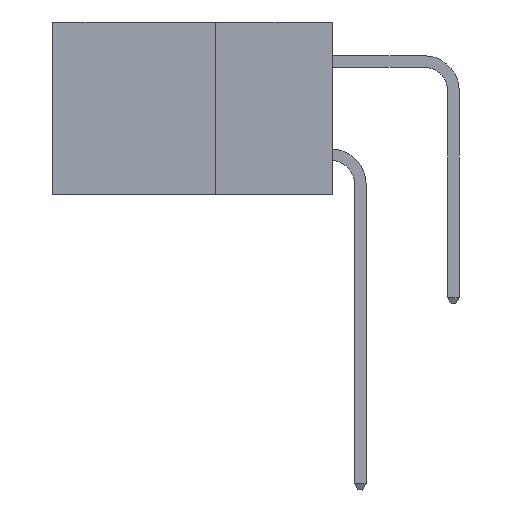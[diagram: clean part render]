
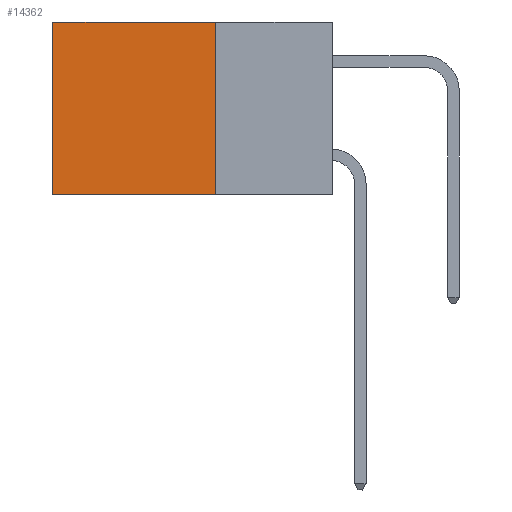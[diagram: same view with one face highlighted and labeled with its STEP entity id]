
A CAD part, left-side view. The second image highlights one B-rep face of the part: STEP entity #14362.
In plain terms, the highlighted planar face has unit normal (-1, 0, 0).
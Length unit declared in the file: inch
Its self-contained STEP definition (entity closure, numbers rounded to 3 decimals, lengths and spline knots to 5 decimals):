
#1033 = LINE ( 'NONE', #18068, #15423 ) ;
#1094 = VERTEX_POINT ( 'NONE', #8958 ) ;
#2006 = AXIS2_PLACEMENT_3D ( 'NONE', #20514, #6875, #14598 ) ;
#4062 = LINE ( 'NONE', #20553, #10786 ) ;
#6875 = DIRECTION ( 'NONE',  ( 1., 0., 0. ) ) ;
#6929 = VERTEX_POINT ( 'NONE', #7179 ) ;
#7179 = CARTESIAN_POINT ( 'NONE',  ( 0.298, 0.25, 0. ) ) ;
#7870 = DIRECTION ( 'NONE',  ( 0., 0., -1. ) ) ;
#8121 = DIRECTION ( 'NONE',  ( 0., 1., 0. ) ) ;
#8219 = ORIENTED_EDGE ( 'NONE', *, *, #24438, .F. ) ;
#8958 = CARTESIAN_POINT ( 'NONE',  ( 0.298, 0.6, -0.37 ) ) ;
#9236 = EDGE_CURVE ( 'NONE', #17482, #1094, #4062, .T. ) ;
#10098 = CARTESIAN_POINT ( 'NONE',  ( 0.298, 0.25, 0. ) ) ;
#10786 = VECTOR ( 'NONE', #18570, 39.37008 ) ;
#12137 = EDGE_CURVE ( 'NONE', #6929, #18030, #25030, .T. ) ;
#12881 = PLANE ( 'NONE',  #2006 ) ;
#14362 = ADVANCED_FACE ( 'NONE', ( #23964 ), #12881, .F. ) ;
#14598 = DIRECTION ( 'NONE',  ( 0., 0., -1. ) ) ;
#14950 = ORIENTED_EDGE ( 'NONE', *, *, #9236, .T. ) ;
#15423 = VECTOR ( 'NONE', #23909, 39.37008 ) ;
#17003 = CARTESIAN_POINT ( 'NONE',  ( 0.298, 0.25, -0.37 ) ) ;
#17482 = VERTEX_POINT ( 'NONE', #20451 ) ;
#17632 = CARTESIAN_POINT ( 'NONE',  ( 0.298, 0.25, 0. ) ) ;
#18030 = VERTEX_POINT ( 'NONE', #17003 ) ;
#18068 = CARTESIAN_POINT ( 'NONE',  ( 0.298, 0.25, -0.37 ) ) ;
#18090 = LINE ( 'NONE', #10098, #18379 ) ;
#18379 = VECTOR ( 'NONE', #8121, 39.37008 ) ;
#18535 = ORIENTED_EDGE ( 'NONE', *, *, #12137, .F. ) ;
#18570 = DIRECTION ( 'NONE',  ( 0., 0., -1. ) ) ;
#19507 = VECTOR ( 'NONE', #7870, 39.37008 ) ;
#19540 = EDGE_CURVE ( 'NONE', #6929, #17482, #18090, .T. ) ;
#20451 = CARTESIAN_POINT ( 'NONE',  ( 0.298, 0.6, 0. ) ) ;
#20514 = CARTESIAN_POINT ( 'NONE',  ( 0.298, 0.25, 0. ) ) ;
#20553 = CARTESIAN_POINT ( 'NONE',  ( 0.298, 0.6, 0. ) ) ;
#23909 = DIRECTION ( 'NONE',  ( 0., 1., 0. ) ) ;
#23964 = FACE_OUTER_BOUND ( 'NONE', #24897, .T. ) ;
#24056 = ORIENTED_EDGE ( 'NONE', *, *, #19540, .T. ) ;
#24438 = EDGE_CURVE ( 'NONE', #18030, #1094, #1033, .T. ) ;
#24897 = EDGE_LOOP ( 'NONE', ( #14950, #8219, #18535, #24056 ) ) ;
#25030 = LINE ( 'NONE', #17632, #19507 ) ;
